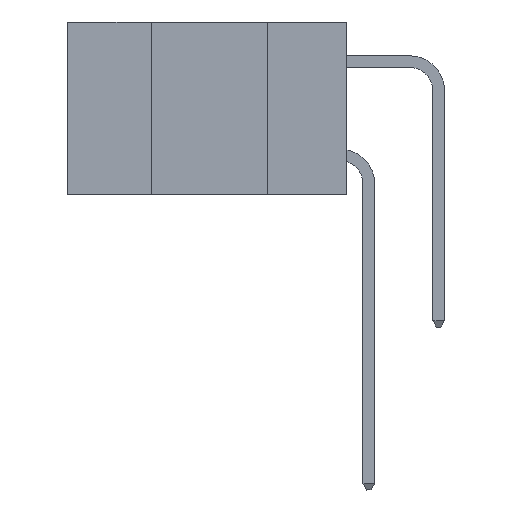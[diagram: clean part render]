
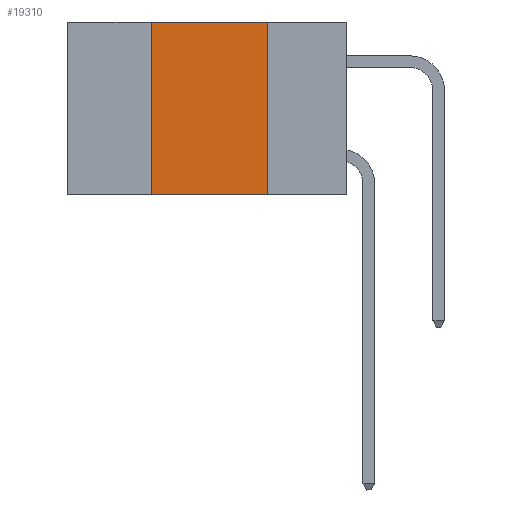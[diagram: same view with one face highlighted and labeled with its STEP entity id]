
A CAD part, left-side view. The second image highlights one B-rep face of the part: STEP entity #19310.
In plain terms, the highlighted planar face has unit normal (-1, 0, 0).
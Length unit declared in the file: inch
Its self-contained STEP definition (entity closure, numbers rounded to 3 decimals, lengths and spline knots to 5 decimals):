
#684 = ORIENTED_EDGE ( 'NONE', *, *, #13000, .F. ) ;
#1249 = VERTEX_POINT ( 'NONE', #11276 ) ;
#2314 = DIRECTION ( 'NONE',  ( 0., 0., -1. ) ) ;
#3736 = FACE_OUTER_BOUND ( 'NONE', #4472, .T. ) ;
#4005 = VERTEX_POINT ( 'NONE', #12576 ) ;
#4472 = EDGE_LOOP ( 'NONE', ( #13751, #21352, #684, #8348 ) ) ;
#6124 = VECTOR ( 'NONE', #11756, 39.37008 ) ;
#6586 = CARTESIAN_POINT ( 'NONE',  ( 0., 0.42, 0. ) ) ;
#7112 = VERTEX_POINT ( 'NONE', #17611 ) ;
#7602 = EDGE_CURVE ( 'NONE', #4005, #1249, #10454, .T. ) ;
#8133 = VECTOR ( 'NONE', #10167, 39.37008 ) ;
#8348 = ORIENTED_EDGE ( 'NONE', *, *, #7602, .T. ) ;
#9519 = DIRECTION ( 'NONE',  ( 0., -1., 0. ) ) ;
#9769 = PLANE ( 'NONE',  #12045 ) ;
#9949 = VECTOR ( 'NONE', #17487, 39.37008 ) ;
#10167 = DIRECTION ( 'NONE',  ( 0., 0., -1. ) ) ;
#10288 = LINE ( 'NONE', #20260, #19311 ) ;
#10454 = LINE ( 'NONE', #20721, #6124 ) ;
#11276 = CARTESIAN_POINT ( 'NONE',  ( 0., 0.17, -0.37 ) ) ;
#11603 = CARTESIAN_POINT ( 'NONE',  ( 0., 0.6, 0. ) ) ;
#11756 = DIRECTION ( 'NONE',  ( 0., -1., 0. ) ) ;
#12045 = AXIS2_PLACEMENT_3D ( 'NONE', #11603, #13446, #2314 ) ;
#12576 = CARTESIAN_POINT ( 'NONE',  ( 0., 0.42, -0.37 ) ) ;
#13000 = EDGE_CURVE ( 'NONE', #4005, #14564, #19534, .T. ) ;
#13446 = DIRECTION ( 'NONE',  ( 1., 0., 0. ) ) ;
#13751 = ORIENTED_EDGE ( 'NONE', *, *, #19445, .F. ) ;
#14564 = VERTEX_POINT ( 'NONE', #19979 ) ;
#17487 = DIRECTION ( 'NONE',  ( 0., 0., 1. ) ) ;
#17611 = CARTESIAN_POINT ( 'NONE',  ( 0., 0.17, 0. ) ) ;
#18375 = LINE ( 'NONE', #19150, #8133 ) ;
#19150 = CARTESIAN_POINT ( 'NONE',  ( 0., 0.17, 0. ) ) ;
#19310 = ADVANCED_FACE ( 'NONE', ( #3736 ), #9769, .F. ) ;
#19311 = VECTOR ( 'NONE', #9519, 39.37008 ) ;
#19445 = EDGE_CURVE ( 'NONE', #7112, #1249, #18375, .T. ) ;
#19534 = LINE ( 'NONE', #6586, #9949 ) ;
#19979 = CARTESIAN_POINT ( 'NONE',  ( 0., 0.42, 0. ) ) ;
#20260 = CARTESIAN_POINT ( 'NONE',  ( 0., 0.6, 0. ) ) ;
#20721 = CARTESIAN_POINT ( 'NONE',  ( 0., 0.6, -0.37 ) ) ;
#21352 = ORIENTED_EDGE ( 'NONE', *, *, #23436, .F. ) ;
#23436 = EDGE_CURVE ( 'NONE', #14564, #7112, #10288, .T. ) ;
